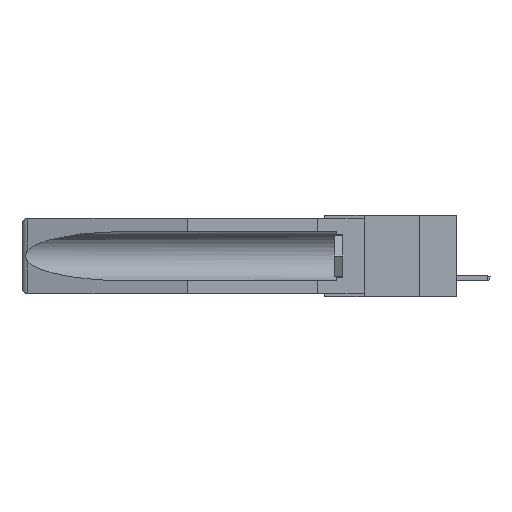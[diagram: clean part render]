
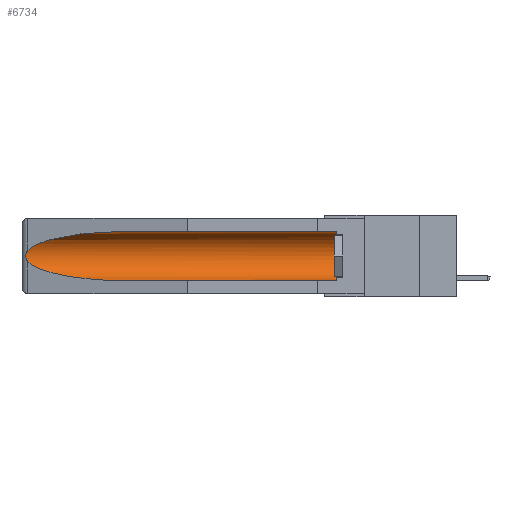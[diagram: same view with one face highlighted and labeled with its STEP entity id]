
A CAD part, left-side view. The second image highlights one B-rep face of the part: STEP entity #6734.
In plain terms, the highlighted cylindrical face has radius 2.857 mm (diameter 5.715 mm), a partial arc.
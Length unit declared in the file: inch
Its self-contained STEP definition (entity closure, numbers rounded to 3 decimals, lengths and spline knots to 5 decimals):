
#7 = VERTEX_POINT ( 'NONE', #877 ) ;
#814 = AXIS2_PLACEMENT_3D ( 'NONE', #14465, #3234, #1891 ) ;
#877 = CARTESIAN_POINT ( 'NONE',  ( 0.155, 1.07973, -0.059 ) ) ;
#895 = VECTOR ( 'NONE', #2026, 39.37008 ) ;
#955 = VERTEX_POINT ( 'NONE', #17649 ) ;
#1045 = ORIENTED_EDGE ( 'NONE', *, *, #2640, .T. ) ;
#1403 = EDGE_CURVE ( 'NONE', #955, #7, #16948, .T. ) ;
#1891 = DIRECTION ( 'NONE',  ( 0., 0., 1. ) ) ;
#1964 = CARTESIAN_POINT ( 'NONE',  ( 0.26537, 1.52718, -0.19328 ) ) ;
#2026 = DIRECTION ( 'NONE',  ( 0., 1., 0. ) ) ;
#2640 = EDGE_CURVE ( 'NONE', #9540, #5782, #6889, .T. ) ;
#3234 = DIRECTION ( 'NONE',  ( 0., 1., 0. ) ) ;
#3253 = CARTESIAN_POINT ( 'NONE',  ( 0.26654, 1.53092, -0.15636 ) ) ;
#3427 = ORIENTED_EDGE ( 'NONE', *, *, #16182, .F. ) ;
#3433 = CARTESIAN_POINT ( 'NONE',  ( 0.2675, 1.53308, -0.16763 ) ) ;
#3645 = CARTESIAN_POINT ( 'NONE',  ( 0.26537, 1.52718, -0.14972 ) ) ;
#4321 = EDGE_CURVE ( 'NONE', #7, #9540, #14580, .T. ) ;
#4441 = EDGE_CURVE ( 'NONE', #4712, #955, #9121, .T. ) ;
#4664 = CARTESIAN_POINT ( 'NONE',  ( 0.26655, 1.53094, -0.18657 ) ) ;
#4712 = VERTEX_POINT ( 'NONE', #12554 ) ;
#5782 = VERTEX_POINT ( 'NONE', #9554 ) ;
#5783 = CARTESIAN_POINT ( 'NONE',  ( 0.25451, 1.48313, -0.24835 ) ) ;
#6146 = CARTESIAN_POINT ( 'NONE',  ( 0.26537, 1.52718, -0.14972 ) ) ;
#6331 = CARTESIAN_POINT ( 'NONE',  ( 0.26597, 1.52961, -0.15275 ) ) ;
#6421 = ORIENTED_EDGE ( 'NONE', *, *, #8753, .T. ) ;
#6422 = DIRECTION ( 'NONE',  ( 0., 0., 1. ) ) ;
#6734 = ADVANCED_FACE ( 'NONE', ( #14707 ), #7102, .F. ) ;
#6817 = DIRECTION ( 'NONE',  ( 0., 1., 0. ) ) ;
#6824 = CARTESIAN_POINT ( 'NONE',  ( 0.21114, 1.30732, -0.059 ) ) ;
#6878 = VECTOR ( 'NONE', #6817, 39.37008 ) ;
#6889 = B_SPLINE_CURVE_WITH_KNOTS ( 'NONE', 3,
 ( #6146, #6331, #3253, #7726, #3433, #13166, #11748, #4664, #17548, #1964 ),
 .UNSPECIFIED., .F., .F.,
 ( 4, 2, 2, 2, 4 ),
 ( 0., 0.00029, 0.00058, 0.00087, 0.00117 ),
 .UNSPECIFIED. ) ;
#7102 = CYLINDRICAL_SURFACE ( 'NONE', #814, 0.1125 ) ;
#7119 =( BOUNDED_CURVE ( )  B_SPLINE_CURVE ( 3, ( #15603, #5783, #17246, #14387 ),
 .UNSPECIFIED., .F., .F. ) 
 B_SPLINE_CURVE_WITH_KNOTS ( ( 4, 4 ),
 ( 0.1948, 1.5708 ),
 .UNSPECIFIED. ) 
 CURVE ( )  GEOMETRIC_REPRESENTATION_ITEM ( )  RATIONAL_B_SPLINE_CURVE ( ( 1., 0.848, 0.848, 1. ) ) 
 REPRESENTATION_ITEM ( '' )  );
#7726 = CARTESIAN_POINT ( 'NONE',  ( 0.2673, 1.5327, -0.16383 ) ) ;
#8247 = CARTESIAN_POINT ( 'NONE',  ( 0.26537, 1.52718, -0.14972 ) ) ;
#8303 = ORIENTED_EDGE ( 'NONE', *, *, #4321, .T. ) ;
#8438 = EDGE_LOOP ( 'NONE', ( #8303, #1045, #6421, #3427, #9026, #15589 ) ) ;
#8753 = EDGE_CURVE ( 'NONE', #5782, #12687, #7119, .T. ) ;
#9026 = ORIENTED_EDGE ( 'NONE', *, *, #4441, .T. ) ;
#9087 = CARTESIAN_POINT ( 'NONE',  ( 0.155, -0.30754, -0.059 ) ) ;
#9121 = CIRCLE ( 'NONE', #12588, 0.1125 ) ;
#9540 = VERTEX_POINT ( 'NONE', #3645 ) ;
#9554 = CARTESIAN_POINT ( 'NONE',  ( 0.26537, 1.52718, -0.19328 ) ) ;
#10659 = DIRECTION ( 'NONE',  ( 0., -1., 0. ) ) ;
#10848 = CARTESIAN_POINT ( 'NONE',  ( 0.155, 0.126, -0.1715 ) ) ;
#11748 = CARTESIAN_POINT ( 'NONE',  ( 0.2673, 1.53269, -0.17917 ) ) ;
#12005 = LINE ( 'NONE', #12454, #6878 ) ;
#12454 = CARTESIAN_POINT ( 'NONE',  ( 0.155, -0.30754, -0.284 ) ) ;
#12554 = CARTESIAN_POINT ( 'NONE',  ( 0.155, 0.126, -0.284 ) ) ;
#12564 = CARTESIAN_POINT ( 'NONE',  ( 0.155, 1.07973, -0.284 ) ) ;
#12588 = AXIS2_PLACEMENT_3D ( 'NONE', #10848, #10659, #6422 ) ;
#12687 = VERTEX_POINT ( 'NONE', #12564 ) ;
#13166 = CARTESIAN_POINT ( 'NONE',  ( 0.2675, 1.53308, -0.17534 ) ) ;
#14387 = CARTESIAN_POINT ( 'NONE',  ( 0.155, 1.07973, -0.284 ) ) ;
#14465 = CARTESIAN_POINT ( 'NONE',  ( 0.155, -0.30754, -0.1715 ) ) ;
#14580 =( BOUNDED_CURVE ( )  B_SPLINE_CURVE ( 3, ( #15354, #6824, #16908, #8247 ),
 .UNSPECIFIED., .F., .F. ) 
 B_SPLINE_CURVE_WITH_KNOTS ( ( 4, 4 ),
 ( 4.71239, 6.08839 ),
 .UNSPECIFIED. ) 
 CURVE ( )  GEOMETRIC_REPRESENTATION_ITEM ( )  RATIONAL_B_SPLINE_CURVE ( ( 1., 0.848, 0.848, 1. ) ) 
 REPRESENTATION_ITEM ( '' )  );
#14707 = FACE_OUTER_BOUND ( 'NONE', #8438, .T. ) ;
#15354 = CARTESIAN_POINT ( 'NONE',  ( 0.155, 1.07973, -0.059 ) ) ;
#15589 = ORIENTED_EDGE ( 'NONE', *, *, #1403, .T. ) ;
#15603 = CARTESIAN_POINT ( 'NONE',  ( 0.26537, 1.52718, -0.19328 ) ) ;
#16182 = EDGE_CURVE ( 'NONE', #4712, #12687, #12005, .T. ) ;
#16908 = CARTESIAN_POINT ( 'NONE',  ( 0.25451, 1.48313, -0.09465 ) ) ;
#16948 = LINE ( 'NONE', #9087, #895 ) ;
#17246 = CARTESIAN_POINT ( 'NONE',  ( 0.21114, 1.30732, -0.284 ) ) ;
#17548 = CARTESIAN_POINT ( 'NONE',  ( 0.26597, 1.5296, -0.19026 ) ) ;
#17649 = CARTESIAN_POINT ( 'NONE',  ( 0.155, 0.126, -0.059 ) ) ;
